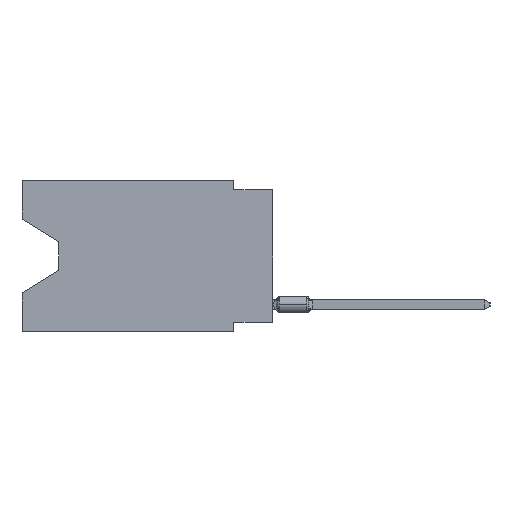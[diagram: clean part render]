
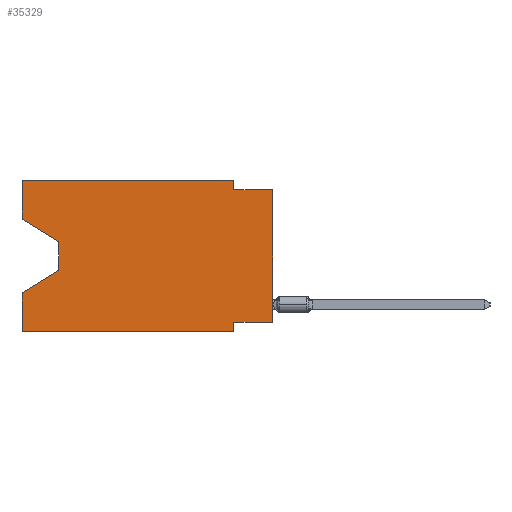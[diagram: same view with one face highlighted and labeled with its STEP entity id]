
A CAD part, left-side view. The second image highlights one B-rep face of the part: STEP entity #35329.
In plain terms, the highlighted planar face has unit normal (-1, 0, 0).
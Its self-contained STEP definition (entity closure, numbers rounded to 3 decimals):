
#740 = VECTOR ( 'NONE', #7557, 1000. ) ;
#1767 = LINE ( 'NONE', #36649, #43470 ) ;
#4253 = VERTEX_POINT ( 'NONE', #30787 ) ;
#5206 = VECTOR ( 'NONE', #28609, 1000. ) ;
#6324 = CARTESIAN_POINT ( 'NONE',  ( 0., 0., -9.271 ) ) ;
#6595 = CARTESIAN_POINT ( 'NONE',  ( 0., 2.54, 0. ) ) ;
#7557 = DIRECTION ( 'NONE',  ( 0., -1., 0. ) ) ;
#10977 = LINE ( 'NONE', #40486, #5206 ) ;
#13436 = CARTESIAN_POINT ( 'NONE',  ( 0., 13.97, -4.013 ) ) ;
#13799 = ORIENTED_EDGE ( 'NONE', *, *, #16557, .F. ) ;
#14474 = DIRECTION ( 'NONE',  ( 0., 0., -1. ) ) ;
#16557 = EDGE_CURVE ( 'NONE', #48051, #30470, #74769, .T. ) ;
#17445 = VECTOR ( 'NONE', #40221, 1000. ) ;
#18387 = VERTEX_POINT ( 'NONE', #74559 ) ;
#18562 = VERTEX_POINT ( 'NONE', #60283 ) ;
#19498 = CARTESIAN_POINT ( 'NONE',  ( 0., 16.383, -2.546 ) ) ;
#19835 = DIRECTION ( 'NONE',  ( 1., 0., 0. ) ) ;
#19936 = VERTEX_POINT ( 'NONE', #6595 ) ;
#20016 = LINE ( 'NONE', #48774, #50990 ) ;
#20452 = LINE ( 'NONE', #41662, #32533 ) ;
#22928 = ORIENTED_EDGE ( 'NONE', *, *, #43770, .T. ) ;
#22977 = DIRECTION ( 'NONE',  ( 0., -1., 0. ) ) ;
#24778 = ORIENTED_EDGE ( 'NONE', *, *, #72471, .F. ) ;
#27877 = EDGE_CURVE ( 'NONE', #30774, #18562, #20452, .T. ) ;
#28609 = DIRECTION ( 'NONE',  ( 0., 0., -1. ) ) ;
#29077 = EDGE_CURVE ( 'NONE', #32567, #37738, #1767, .T. ) ;
#30470 = VERTEX_POINT ( 'NONE', #31146 ) ;
#30774 = VERTEX_POINT ( 'NONE', #13436 ) ;
#30787 = CARTESIAN_POINT ( 'NONE',  ( 0., 0., -0.635 ) ) ;
#30952 = CARTESIAN_POINT ( 'NONE',  ( 0., 2.54, 0. ) ) ;
#31146 = CARTESIAN_POINT ( 'NONE',  ( 0., 16.383, -7.36 ) ) ;
#32533 = VECTOR ( 'NONE', #73332, 1000. ) ;
#32567 = VERTEX_POINT ( 'NONE', #19498 ) ;
#34608 = VERTEX_POINT ( 'NONE', #37755 ) ;
#34678 = VECTOR ( 'NONE', #57570, 1000. ) ;
#35329 = ADVANCED_FACE ( 'NONE', ( #75587 ), #66595, .F. ) ;
#35330 = EDGE_CURVE ( 'NONE', #19936, #42759, #66224, .T. ) ;
#36649 = CARTESIAN_POINT ( 'NONE',  ( 0., 16.383, 0. ) ) ;
#36931 = ORIENTED_EDGE ( 'NONE', *, *, #27877, .T. ) ;
#37738 = VERTEX_POINT ( 'NONE', #69867 ) ;
#37755 = CARTESIAN_POINT ( 'NONE',  ( 0., 0., -9.271 ) ) ;
#39078 = LINE ( 'NONE', #55967, #61576 ) ;
#39150 = VECTOR ( 'NONE', #75735, 1000. ) ;
#39151 = EDGE_CURVE ( 'NONE', #48051, #71786, #52210, .T. ) ;
#39882 = CARTESIAN_POINT ( 'NONE',  ( 0., 16.383, 0. ) ) ;
#40221 = DIRECTION ( 'NONE',  ( 0., -0.855, -0.519 ) ) ;
#40263 = DIRECTION ( 'NONE',  ( 0., 0., 1. ) ) ;
#40486 = CARTESIAN_POINT ( 'NONE',  ( 0., 2.54, -9.906 ) ) ;
#40740 = ORIENTED_EDGE ( 'NONE', *, *, #46032, .T. ) ;
#40839 = LINE ( 'NONE', #6324, #39150 ) ;
#41662 = CARTESIAN_POINT ( 'NONE',  ( 0., 13.97, -4.013 ) ) ;
#42091 = VECTOR ( 'NONE', #22977, 1000. ) ;
#42465 = CARTESIAN_POINT ( 'NONE',  ( 0., 16.383, 0. ) ) ;
#42759 = VERTEX_POINT ( 'NONE', #60061 ) ;
#42856 = CARTESIAN_POINT ( 'NONE',  ( 0., 16.383, 0. ) ) ;
#43380 = ORIENTED_EDGE ( 'NONE', *, *, #67428, .F. ) ;
#43470 = VECTOR ( 'NONE', #48923, 1000. ) ;
#43522 = CARTESIAN_POINT ( 'NONE',  ( 0., 16.383, -9.906 ) ) ;
#43690 = DIRECTION ( 'NONE',  ( 0., 0., 1. ) ) ;
#43770 = EDGE_CURVE ( 'NONE', #32567, #30774, #63592, .T. ) ;
#45445 = EDGE_CURVE ( 'NONE', #42759, #4253, #75496, .T. ) ;
#46032 = EDGE_CURVE ( 'NONE', #34608, #4253, #39078, .T. ) ;
#47043 = AXIS2_PLACEMENT_3D ( 'NONE', #42856, #19835, #14474 ) ;
#47198 = DIRECTION ( 'NONE',  ( 0., 0., -1. ) ) ;
#48051 = VERTEX_POINT ( 'NONE', #43522 ) ;
#48774 = CARTESIAN_POINT ( 'NONE',  ( 0., 13.97, -5.893 ) ) ;
#48851 = EDGE_LOOP ( 'NONE', ( #22928, #36931, #53133, #13799, #63256, #24778, #71012, #40740, #51191, #75361, #43380, #54322 ) ) ;
#48923 = DIRECTION ( 'NONE',  ( 0., 0., 1. ) ) ;
#50763 = VECTOR ( 'NONE', #40263, 1000. ) ;
#50990 = VECTOR ( 'NONE', #66405, 1000. ) ;
#51191 = ORIENTED_EDGE ( 'NONE', *, *, #45445, .F. ) ;
#52210 = LINE ( 'NONE', #75585, #34678 ) ;
#53133 = ORIENTED_EDGE ( 'NONE', *, *, #55909, .T. ) ;
#54322 = ORIENTED_EDGE ( 'NONE', *, *, #29077, .F. ) ;
#55909 = EDGE_CURVE ( 'NONE', #18562, #30470, #20016, .T. ) ;
#55967 = CARTESIAN_POINT ( 'NONE',  ( 0., 0., 0. ) ) ;
#57570 = DIRECTION ( 'NONE',  ( 0., -1., 0. ) ) ;
#59291 = EDGE_CURVE ( 'NONE', #34608, #18387, #40839, .T. ) ;
#60061 = CARTESIAN_POINT ( 'NONE',  ( 0., 2.54, -0.635 ) ) ;
#60283 = CARTESIAN_POINT ( 'NONE',  ( 0., 13.97, -5.893 ) ) ;
#61576 = VECTOR ( 'NONE', #43690, 1000. ) ;
#63234 = CARTESIAN_POINT ( 'NONE',  ( 0., 0., -0.635 ) ) ;
#63256 = ORIENTED_EDGE ( 'NONE', *, *, #39151, .T. ) ;
#63592 = LINE ( 'NONE', #68967, #17445 ) ;
#66224 = LINE ( 'NONE', #30952, #72696 ) ;
#66405 = DIRECTION ( 'NONE',  ( 0., 0.855, -0.519 ) ) ;
#66595 = PLANE ( 'NONE',  #47043 ) ;
#67428 = EDGE_CURVE ( 'NONE', #37738, #19936, #73104, .T. ) ;
#68967 = CARTESIAN_POINT ( 'NONE',  ( 0., 16.383, -2.546 ) ) ;
#69867 = CARTESIAN_POINT ( 'NONE',  ( 0., 16.383, 0. ) ) ;
#70570 = CARTESIAN_POINT ( 'NONE',  ( 0., 2.54, -9.906 ) ) ;
#71012 = ORIENTED_EDGE ( 'NONE', *, *, #59291, .F. ) ;
#71786 = VERTEX_POINT ( 'NONE', #70570 ) ;
#72471 = EDGE_CURVE ( 'NONE', #18387, #71786, #10977, .T. ) ;
#72696 = VECTOR ( 'NONE', #47198, 1000. ) ;
#73104 = LINE ( 'NONE', #42465, #740 ) ;
#73332 = DIRECTION ( 'NONE',  ( 0., 0., -1. ) ) ;
#74559 = CARTESIAN_POINT ( 'NONE',  ( 0., 2.54, -9.271 ) ) ;
#74769 = LINE ( 'NONE', #39882, #50763 ) ;
#75361 = ORIENTED_EDGE ( 'NONE', *, *, #35330, .F. ) ;
#75496 = LINE ( 'NONE', #63234, #42091 ) ;
#75585 = CARTESIAN_POINT ( 'NONE',  ( 0., 16.383, -9.906 ) ) ;
#75587 = FACE_OUTER_BOUND ( 'NONE', #48851, .T. ) ;
#75735 = DIRECTION ( 'NONE',  ( 0., 1., 0. ) ) ;
